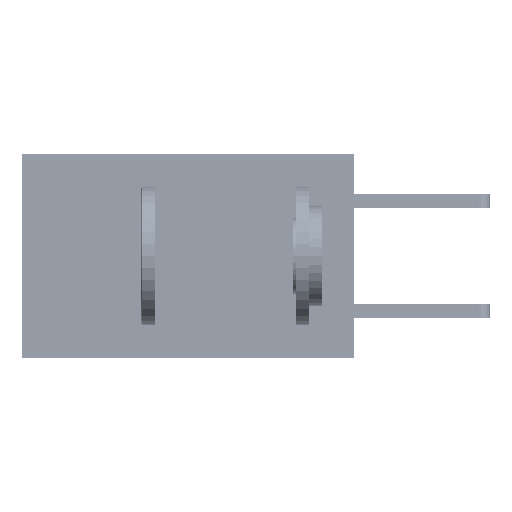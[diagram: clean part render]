
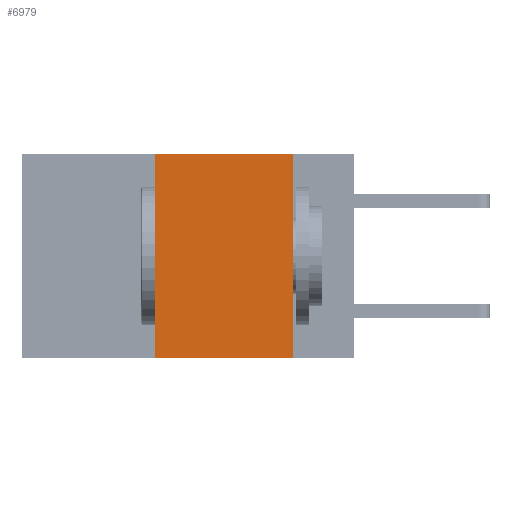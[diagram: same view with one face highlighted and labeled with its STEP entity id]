
A CAD part, left-side view. The second image highlights one B-rep face of the part: STEP entity #6979.
In plain terms, the highlighted planar face has unit normal (-1, 0, 0).
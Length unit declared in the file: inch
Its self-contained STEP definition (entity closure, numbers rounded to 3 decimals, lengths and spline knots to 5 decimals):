
#625 = VERTEX_POINT ( 'NONE', #41832 ) ;
#2586 = VECTOR ( 'NONE', #9959, 39.37008 ) ;
#2678 = EDGE_CURVE ( 'NONE', #625, #42816, #26267, .T. ) ;
#3645 = PLANE ( 'NONE',  #30668 ) ;
#5749 = CARTESIAN_POINT ( 'NONE',  ( 0., 0.6, 0. ) ) ;
#6522 = VERTEX_POINT ( 'NONE', #49572 ) ;
#6824 = DIRECTION ( 'NONE',  ( 0., 0., -1. ) ) ;
#6839 = EDGE_CURVE ( 'NONE', #6522, #36329, #21203, .T. ) ;
#6979 = ADVANCED_FACE ( 'NONE', ( #13735 ), #3645, .F. ) ;
#8393 = DIRECTION ( 'NONE',  ( 1., 0., 0. ) ) ;
#9959 = DIRECTION ( 'NONE',  ( 0., -1., 0. ) ) ;
#11529 = DIRECTION ( 'NONE',  ( 0., -1., 0. ) ) ;
#13735 = FACE_OUTER_BOUND ( 'NONE', #13991, .T. ) ;
#13991 = EDGE_LOOP ( 'NONE', ( #28755, #28850, #23417, #37389 ) ) ;
#17974 = DIRECTION ( 'NONE',  ( 0., 0., 1. ) ) ;
#20427 = EDGE_CURVE ( 'NONE', #42816, #6522, #33916, .T. ) ;
#21203 = LINE ( 'NONE', #51468, #47509 ) ;
#23417 = ORIENTED_EDGE ( 'NONE', *, *, #2678, .F. ) ;
#23980 = DIRECTION ( 'NONE',  ( 0., 0., -1. ) ) ;
#24974 = CARTESIAN_POINT ( 'NONE',  ( 0., 0.11, -0.37 ) ) ;
#26267 = LINE ( 'NONE', #45633, #27512 ) ;
#27512 = VECTOR ( 'NONE', #17974, 39.37008 ) ;
#28755 = ORIENTED_EDGE ( 'NONE', *, *, #6839, .F. ) ;
#28850 = ORIENTED_EDGE ( 'NONE', *, *, #20427, .F. ) ;
#29852 = LINE ( 'NONE', #35468, #31099 ) ;
#30668 = AXIS2_PLACEMENT_3D ( 'NONE', #31610, #8393, #23980 ) ;
#31099 = VECTOR ( 'NONE', #11529, 39.37008 ) ;
#31610 = CARTESIAN_POINT ( 'NONE',  ( 0., 0.6, 0. ) ) ;
#33916 = LINE ( 'NONE', #5749, #2586 ) ;
#35468 = CARTESIAN_POINT ( 'NONE',  ( 0., 0.6, -0.37 ) ) ;
#36329 = VERTEX_POINT ( 'NONE', #24974 ) ;
#37389 = ORIENTED_EDGE ( 'NONE', *, *, #46971, .T. ) ;
#41832 = CARTESIAN_POINT ( 'NONE',  ( 0., 0.36, -0.37 ) ) ;
#42816 = VERTEX_POINT ( 'NONE', #44228 ) ;
#44228 = CARTESIAN_POINT ( 'NONE',  ( 0., 0.36, 0. ) ) ;
#45633 = CARTESIAN_POINT ( 'NONE',  ( 0., 0.36, 0. ) ) ;
#46971 = EDGE_CURVE ( 'NONE', #625, #36329, #29852, .T. ) ;
#47509 = VECTOR ( 'NONE', #6824, 39.37008 ) ;
#49572 = CARTESIAN_POINT ( 'NONE',  ( 0., 0.11, 0. ) ) ;
#51468 = CARTESIAN_POINT ( 'NONE',  ( 0., 0.11, 0. ) ) ;
